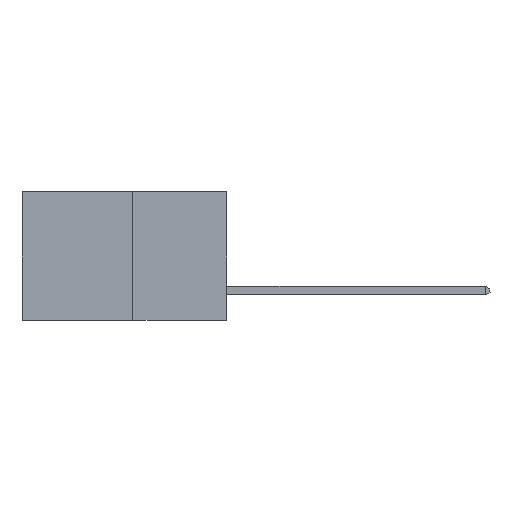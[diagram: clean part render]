
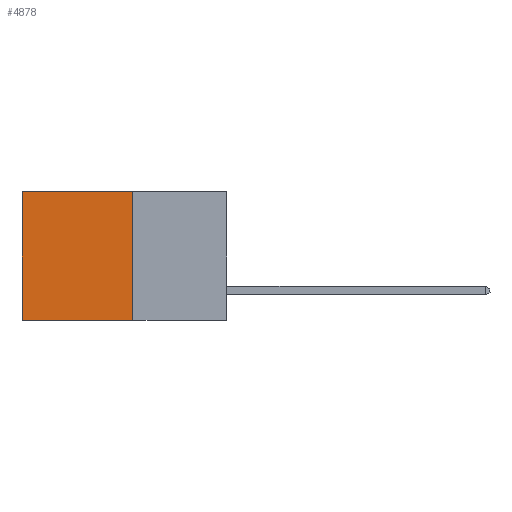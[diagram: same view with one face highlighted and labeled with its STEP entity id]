
A CAD part, left-side view. The second image highlights one B-rep face of the part: STEP entity #4878.
In plain terms, the highlighted planar face has unit normal (-1, 0, 0).
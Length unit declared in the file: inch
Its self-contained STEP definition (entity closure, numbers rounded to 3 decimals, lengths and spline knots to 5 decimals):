
#255 = FACE_OUTER_BOUND ( 'NONE', #5314, .T. ) ;
#431 = CARTESIAN_POINT ( 'NONE',  ( 0.277, 0.59, -0.37 ) ) ;
#497 = DIRECTION ( 'NONE',  ( 0., 1., 0. ) ) ;
#622 = VECTOR ( 'NONE', #497, 39.37008 ) ;
#2558 = EDGE_CURVE ( 'NONE', #2992, #2728, #7774, .T. ) ;
#2728 = VERTEX_POINT ( 'NONE', #431 ) ;
#2992 = VERTEX_POINT ( 'NONE', #9424 ) ;
#3377 = LINE ( 'NONE', #10520, #5485 ) ;
#3658 = LINE ( 'NONE', #10447, #5479 ) ;
#4397 = EDGE_CURVE ( 'NONE', #4540, #2728, #3658, .T. ) ;
#4540 = VERTEX_POINT ( 'NONE', #6442 ) ;
#4661 = AXIS2_PLACEMENT_3D ( 'NONE', #10611, #10410, #10315 ) ;
#4878 = ADVANCED_FACE ( 'NONE', ( #255 ), #10369, .F. ) ;
#5267 = CARTESIAN_POINT ( 'NONE',  ( 0.277, 0.27, 0. ) ) ;
#5314 = EDGE_LOOP ( 'NONE', ( #8083, #7263, #9458, #8101 ) ) ;
#5479 = VECTOR ( 'NONE', #10224, 39.37008 ) ;
#5485 = VECTOR ( 'NONE', #6437, 39.37008 ) ;
#5879 = LINE ( 'NONE', #5267, #8380 ) ;
#6437 = DIRECTION ( 'NONE',  ( 0., 0., -1. ) ) ;
#6442 = CARTESIAN_POINT ( 'NONE',  ( 0.277, 0.59, 0. ) ) ;
#7105 = CARTESIAN_POINT ( 'NONE',  ( 0.277, 0.27, -0.37 ) ) ;
#7263 = ORIENTED_EDGE ( 'NONE', *, *, #2558, .F. ) ;
#7411 = EDGE_CURVE ( 'NONE', #10061, #4540, #5879, .T. ) ;
#7644 = EDGE_CURVE ( 'NONE', #10061, #2992, #3377, .T. ) ;
#7774 = LINE ( 'NONE', #7105, #622 ) ;
#8083 = ORIENTED_EDGE ( 'NONE', *, *, #4397, .T. ) ;
#8101 = ORIENTED_EDGE ( 'NONE', *, *, #7411, .T. ) ;
#8380 = VECTOR ( 'NONE', #10994, 39.37008 ) ;
#9424 = CARTESIAN_POINT ( 'NONE',  ( 0.277, 0.27, -0.37 ) ) ;
#9458 = ORIENTED_EDGE ( 'NONE', *, *, #7644, .F. ) ;
#10061 = VERTEX_POINT ( 'NONE', #11127 ) ;
#10224 = DIRECTION ( 'NONE',  ( 0., 0., -1. ) ) ;
#10315 = DIRECTION ( 'NONE',  ( 0., 0., -1. ) ) ;
#10369 = PLANE ( 'NONE',  #4661 ) ;
#10410 = DIRECTION ( 'NONE',  ( 1., 0., 0. ) ) ;
#10447 = CARTESIAN_POINT ( 'NONE',  ( 0.277, 0.59, -0.37 ) ) ;
#10520 = CARTESIAN_POINT ( 'NONE',  ( 0.277, 0.27, -0.37 ) ) ;
#10611 = CARTESIAN_POINT ( 'NONE',  ( 0.277, 0.27, -0.37 ) ) ;
#10994 = DIRECTION ( 'NONE',  ( 0., 1., 0. ) ) ;
#11127 = CARTESIAN_POINT ( 'NONE',  ( 0.277, 0.27, 0. ) ) ;
